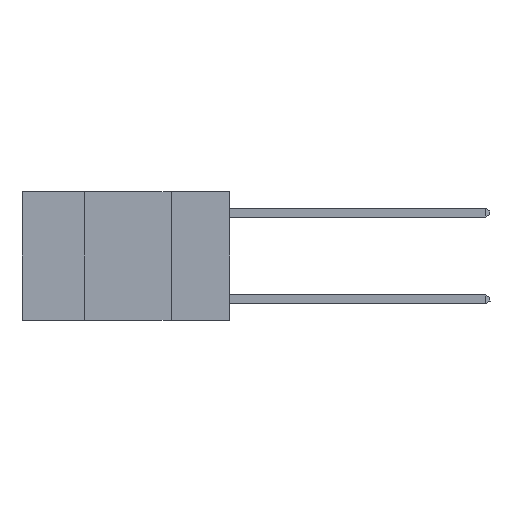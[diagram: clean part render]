
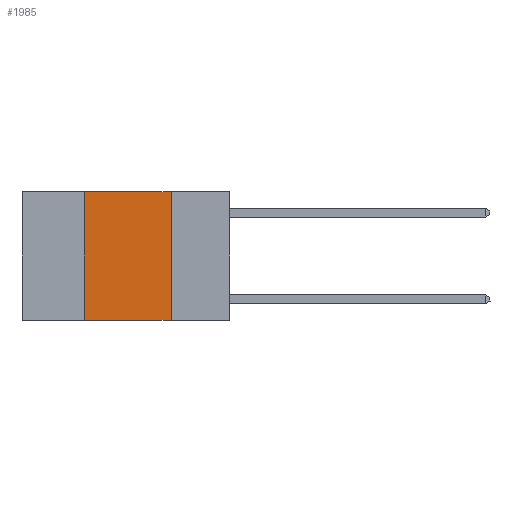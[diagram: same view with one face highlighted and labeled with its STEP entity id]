
A CAD part, left-side view. The second image highlights one B-rep face of the part: STEP entity #1985.
In plain terms, the highlighted planar face has unit normal (-1, 0, 0).
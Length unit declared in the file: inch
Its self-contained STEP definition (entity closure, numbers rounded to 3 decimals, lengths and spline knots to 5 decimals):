
#19 = CARTESIAN_POINT ( 'NONE',  ( 0., 0.42, 0. ) ) ;
#107 = LINE ( 'NONE', #19, #691 ) ;
#691 = VECTOR ( 'NONE', #12498, 39.37008 ) ;
#914 = EDGE_CURVE ( 'NONE', #10725, #6432, #7207, .T. ) ;
#1985 = ADVANCED_FACE ( 'NONE', ( #15844 ), #2019, .F. ) ;
#2019 = PLANE ( 'NONE',  #17775 ) ;
#2177 = CARTESIAN_POINT ( 'NONE',  ( 0., 0.6, 0. ) ) ;
#3827 = CARTESIAN_POINT ( 'NONE',  ( 0., 0.17, 0. ) ) ;
#4010 = LINE ( 'NONE', #8118, #15982 ) ;
#4419 = DIRECTION ( 'NONE',  ( 0., 0., -1. ) ) ;
#6033 = DIRECTION ( 'NONE',  ( 0., 0., -1. ) ) ;
#6432 = VERTEX_POINT ( 'NONE', #8040 ) ;
#6461 = EDGE_CURVE ( 'NONE', #17871, #6432, #4010, .T. ) ;
#7099 = EDGE_LOOP ( 'NONE', ( #7797, #9590, #10998, #16762 ) ) ;
#7207 = LINE ( 'NONE', #9818, #9623 ) ;
#7672 = CARTESIAN_POINT ( 'NONE',  ( 0., 0.42, -0.37 ) ) ;
#7797 = ORIENTED_EDGE ( 'NONE', *, *, #914, .F. ) ;
#7881 = DIRECTION ( 'NONE',  ( 0., -1., 0. ) ) ;
#8040 = CARTESIAN_POINT ( 'NONE',  ( 0., 0.17, -0.37 ) ) ;
#8118 = CARTESIAN_POINT ( 'NONE',  ( 0., 0.6, -0.37 ) ) ;
#8832 = DIRECTION ( 'NONE',  ( 1., 0., 0. ) ) ;
#9590 = ORIENTED_EDGE ( 'NONE', *, *, #14687, .F. ) ;
#9623 = VECTOR ( 'NONE', #4419, 39.37008 ) ;
#9691 = DIRECTION ( 'NONE',  ( 0., -1., 0. ) ) ;
#9818 = CARTESIAN_POINT ( 'NONE',  ( 0., 0.17, 0. ) ) ;
#10374 = EDGE_CURVE ( 'NONE', #17871, #17402, #107, .T. ) ;
#10725 = VERTEX_POINT ( 'NONE', #3827 ) ;
#10998 = ORIENTED_EDGE ( 'NONE', *, *, #10374, .F. ) ;
#12498 = DIRECTION ( 'NONE',  ( 0., 0., 1. ) ) ;
#13101 = CARTESIAN_POINT ( 'NONE',  ( 0., 0.6, 0. ) ) ;
#14687 = EDGE_CURVE ( 'NONE', #17402, #10725, #14960, .T. ) ;
#14960 = LINE ( 'NONE', #2177, #16850 ) ;
#15844 = FACE_OUTER_BOUND ( 'NONE', #7099, .T. ) ;
#15982 = VECTOR ( 'NONE', #9691, 39.37008 ) ;
#16762 = ORIENTED_EDGE ( 'NONE', *, *, #6461, .T. ) ;
#16850 = VECTOR ( 'NONE', #7881, 39.37008 ) ;
#17402 = VERTEX_POINT ( 'NONE', #17850 ) ;
#17775 = AXIS2_PLACEMENT_3D ( 'NONE', #13101, #8832, #6033 ) ;
#17850 = CARTESIAN_POINT ( 'NONE',  ( 0., 0.42, 0. ) ) ;
#17871 = VERTEX_POINT ( 'NONE', #7672 ) ;
